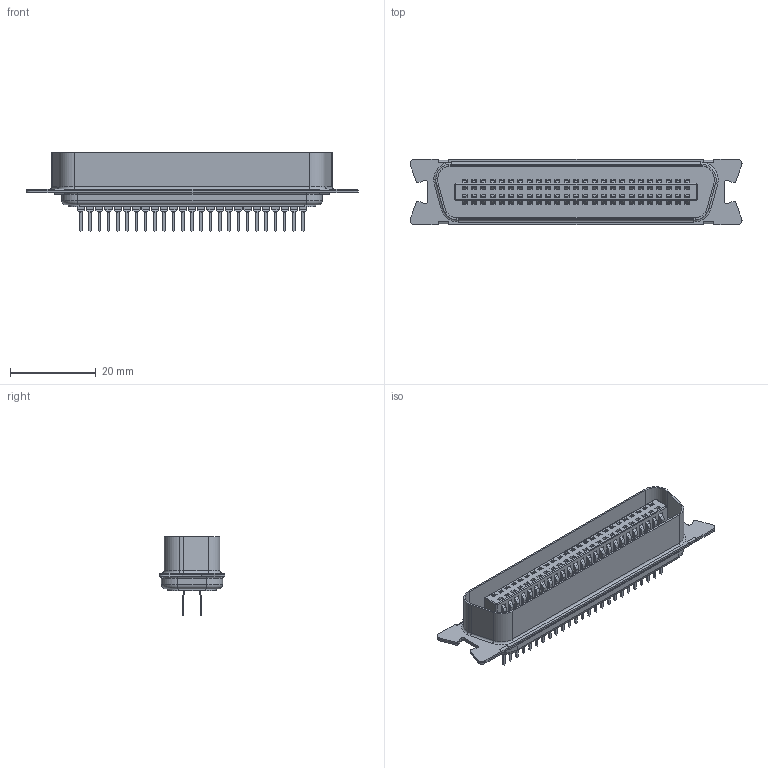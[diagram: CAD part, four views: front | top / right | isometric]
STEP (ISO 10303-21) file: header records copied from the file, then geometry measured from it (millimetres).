
FILE_DESCRIPTION (( 'STEP AP203' ), '1' );
FILE_NAME ('B57-150-621-003.STEP', '2020-06-24T12:29:12', ( '' ), ( '' ), 'SwSTEP 2.0', 'SolidWorks 2020', '' );
FILE_SCHEMA (( 'CONFIG_CONTROL_DESIGN' ));
Length unit declared in the file: millimetre
Products named in the file (5): B57 Back Shell_50 Position LATCH; B57 Front Shell MALE_50 Position LATCH; B57 Contacts MALE_50 Position STR; B57-150-621-003; B57 Housing Insert MALE_50 Position UP
Assembly tree (4 placements, depth 2):
  B57-150-621-003
    B57 Back Shell_50 Position LATCH
    B57 Housing Insert MALE_50 Position UP
    B57 Front Shell MALE_50 Position LATCH
    B57 Contacts MALE_50 Position STR
Bounding box: 77.35 x 15.3 x 18.34 mm (x, y, z)
Volume: 5811.6 mm3; surface area: 14092.7 mm2
Topology: 53 solids, 53 shells, 4864 faces, 13781 edges, 8724 vertices
Faces by surface type: plane 3431, cylinder 1203, sphere 204, torus 26
Entity records: 155298 total; most frequent: CARTESIAN_POINT 29272, ORIENTED_EDGE 27154, DIRECTION 24959, EDGE_CURVE 13577, VECTOR 10937, LINE 10937, VERTEX_POINT 8724, AXIS2_PLACEMENT_3D 7011
